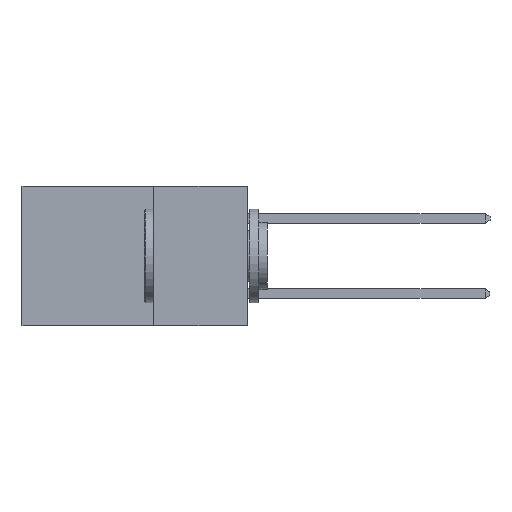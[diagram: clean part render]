
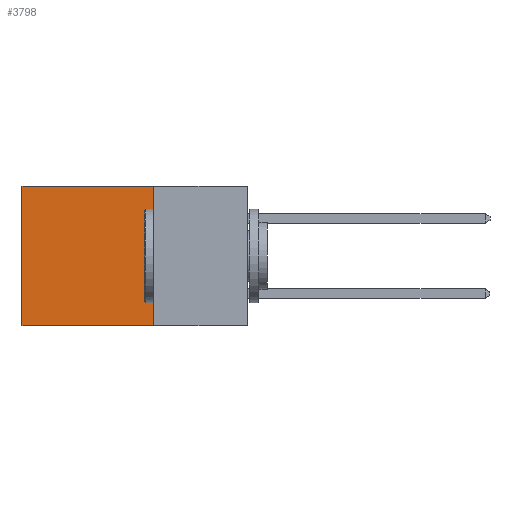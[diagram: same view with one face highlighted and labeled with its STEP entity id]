
A CAD part, left-side view. The second image highlights one B-rep face of the part: STEP entity #3798.
In plain terms, the highlighted planar face has unit normal (-1, 0, 0).
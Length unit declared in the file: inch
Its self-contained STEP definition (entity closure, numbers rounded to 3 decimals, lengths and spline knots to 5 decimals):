
#375 = FACE_OUTER_BOUND ( 'NONE', #15454, .T. ) ;
#801 = DIRECTION ( 'NONE',  ( 0., 0., -1. ) ) ;
#846 = CARTESIAN_POINT ( 'NONE',  ( 0.298, 0.6, 0. ) ) ;
#871 = EDGE_CURVE ( 'NONE', #12861, #14316, #5145, .T. ) ;
#921 = CARTESIAN_POINT ( 'NONE',  ( 0.298, 0.25, 0. ) ) ;
#1140 = ORIENTED_EDGE ( 'NONE', *, *, #12582, .F. ) ;
#1372 = VECTOR ( 'NONE', #801, 39.37008 ) ;
#1611 = VECTOR ( 'NONE', #5062, 39.37008 ) ;
#1754 = VECTOR ( 'NONE', #9582, 39.37008 ) ;
#2987 = CARTESIAN_POINT ( 'NONE',  ( 0.298, 0.6, -0.37 ) ) ;
#3173 = CARTESIAN_POINT ( 'NONE',  ( 0.298, 0.25, 0. ) ) ;
#3266 = EDGE_CURVE ( 'NONE', #14316, #9145, #4216, .T. ) ;
#3798 = ADVANCED_FACE ( 'NONE', ( #375 ), #13753, .F. ) ;
#3826 = CARTESIAN_POINT ( 'NONE',  ( 0.298, 0.25, -0.37 ) ) ;
#4216 = LINE ( 'NONE', #5134, #1611 ) ;
#4943 = EDGE_CURVE ( 'NONE', #12861, #13858, #7997, .T. ) ;
#5062 = DIRECTION ( 'NONE',  ( 0., 0., -1. ) ) ;
#5134 = CARTESIAN_POINT ( 'NONE',  ( 0.298, 0.6, 0. ) ) ;
#5145 = LINE ( 'NONE', #8438, #1754 ) ;
#7029 = ORIENTED_EDGE ( 'NONE', *, *, #4943, .F. ) ;
#7997 = LINE ( 'NONE', #921, #1372 ) ;
#8438 = CARTESIAN_POINT ( 'NONE',  ( 0.298, 0.25, 0. ) ) ;
#9145 = VERTEX_POINT ( 'NONE', #2987 ) ;
#9525 = DIRECTION ( 'NONE',  ( 1., 0., 0. ) ) ;
#9582 = DIRECTION ( 'NONE',  ( 0., 1., 0. ) ) ;
#9832 = DIRECTION ( 'NONE',  ( 0., 0., -1. ) ) ;
#9898 = VECTOR ( 'NONE', #12471, 39.37008 ) ;
#10271 = LINE ( 'NONE', #11234, #9898 ) ;
#10769 = AXIS2_PLACEMENT_3D ( 'NONE', #14964, #9525, #9832 ) ;
#11234 = CARTESIAN_POINT ( 'NONE',  ( 0.298, 0.25, -0.37 ) ) ;
#12036 = ORIENTED_EDGE ( 'NONE', *, *, #3266, .T. ) ;
#12471 = DIRECTION ( 'NONE',  ( 0., 1., 0. ) ) ;
#12528 = ORIENTED_EDGE ( 'NONE', *, *, #871, .T. ) ;
#12582 = EDGE_CURVE ( 'NONE', #13858, #9145, #10271, .T. ) ;
#12861 = VERTEX_POINT ( 'NONE', #3173 ) ;
#13753 = PLANE ( 'NONE',  #10769 ) ;
#13858 = VERTEX_POINT ( 'NONE', #3826 ) ;
#14316 = VERTEX_POINT ( 'NONE', #846 ) ;
#14964 = CARTESIAN_POINT ( 'NONE',  ( 0.298, 0.25, 0. ) ) ;
#15454 = EDGE_LOOP ( 'NONE', ( #12036, #1140, #7029, #12528 ) ) ;
